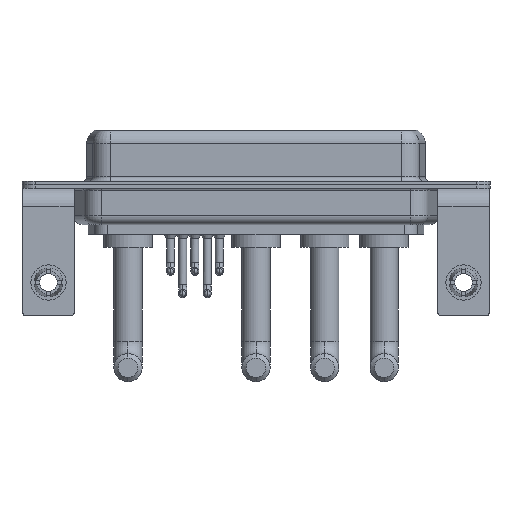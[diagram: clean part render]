
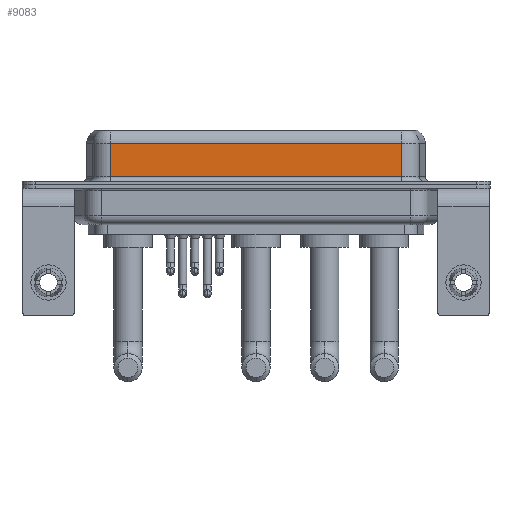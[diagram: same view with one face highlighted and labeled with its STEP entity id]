
A CAD part, front view. The second image highlights one B-rep face of the part: STEP entity #9083.
In plain terms, the highlighted planar face has unit normal (0, -1, 0).
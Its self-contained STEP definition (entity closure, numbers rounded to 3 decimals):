
#664 = EDGE_CURVE ( 'NONE', #10061, #18783, #18149, .T. ) ;
#1715 = DIRECTION ( 'NONE',  ( -1., 0., 0. ) ) ;
#1935 = VERTEX_POINT ( 'NONE', #13731 ) ;
#2194 = CARTESIAN_POINT ( 'NONE',  ( 40.037, -3.95, 0.9 ) ) ;
#2350 = CARTESIAN_POINT ( 'NONE',  ( 40.037, -3.95, 6.4 ) ) ;
#2452 = DIRECTION ( 'NONE',  ( 0., 0., 1. ) ) ;
#2861 = DIRECTION ( 'NONE',  ( 1., 0., 0. ) ) ;
#3148 = VECTOR ( 'NONE', #2861, 1000. ) ;
#3839 = PLANE ( 'NONE',  #8042 ) ;
#3927 = VECTOR ( 'NONE', #1715, 1000. ) ;
#4388 = DIRECTION ( 'NONE',  ( 0., 0., -1. ) ) ;
#5352 = VECTOR ( 'NONE', #19653, 1000. ) ;
#5681 = ORIENTED_EDGE ( 'NONE', *, *, #6422, .T. ) ;
#6422 = EDGE_CURVE ( 'NONE', #10061, #1935, #16817, .T. ) ;
#6910 = ORIENTED_EDGE ( 'NONE', *, *, #664, .F. ) ;
#7444 = CARTESIAN_POINT ( 'NONE',  ( 7.013, -3.95, 6.4 ) ) ;
#7713 = ORIENTED_EDGE ( 'NONE', *, *, #10748, .T. ) ;
#7878 = CARTESIAN_POINT ( 'NONE',  ( 7.013, -3.95, 0.9 ) ) ;
#8042 = AXIS2_PLACEMENT_3D ( 'NONE', #2350, #14850, #2452 ) ;
#9083 = ADVANCED_FACE ( 'NONE', ( #11473 ), #3839, .F. ) ;
#10051 = VERTEX_POINT ( 'NONE', #7878 ) ;
#10061 = VERTEX_POINT ( 'NONE', #12542 ) ;
#10297 = CARTESIAN_POINT ( 'NONE',  ( 40.037, -3.95, 6.4 ) ) ;
#10380 = EDGE_CURVE ( 'NONE', #1935, #10051, #14898, .T. ) ;
#10748 = EDGE_CURVE ( 'NONE', #10051, #18783, #16477, .T. ) ;
#11473 = FACE_OUTER_BOUND ( 'NONE', #17161, .T. ) ;
#12134 = ORIENTED_EDGE ( 'NONE', *, *, #10380, .T. ) ;
#12140 = CARTESIAN_POINT ( 'NONE',  ( 40.037, -3.95, 4.65 ) ) ;
#12283 = VECTOR ( 'NONE', #4388, 1000. ) ;
#12542 = CARTESIAN_POINT ( 'NONE',  ( 40.037, -3.95, 4.65 ) ) ;
#13731 = CARTESIAN_POINT ( 'NONE',  ( 7.013, -3.95, 4.65 ) ) ;
#14850 = DIRECTION ( 'NONE',  ( 0., 1., 0. ) ) ;
#14898 = LINE ( 'NONE', #7444, #12283 ) ;
#16477 = LINE ( 'NONE', #17768, #3148 ) ;
#16817 = LINE ( 'NONE', #12140, #3927 ) ;
#17161 = EDGE_LOOP ( 'NONE', ( #6910, #5681, #12134, #7713 ) ) ;
#17768 = CARTESIAN_POINT ( 'NONE',  ( 40.037, -3.95, 0.9 ) ) ;
#18149 = LINE ( 'NONE', #10297, #5352 ) ;
#18783 = VERTEX_POINT ( 'NONE', #2194 ) ;
#19653 = DIRECTION ( 'NONE',  ( 0., 0., -1. ) ) ;
